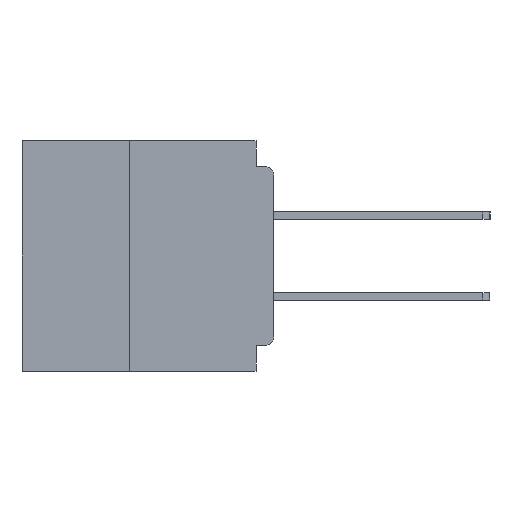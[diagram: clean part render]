
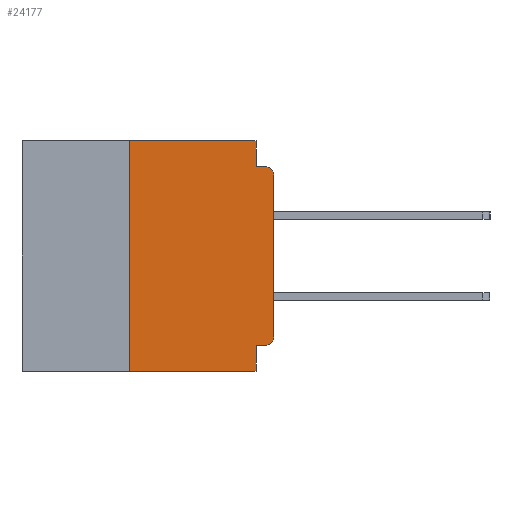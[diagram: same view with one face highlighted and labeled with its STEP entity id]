
A CAD part, left-side view. The second image highlights one B-rep face of the part: STEP entity #24177.
In plain terms, the highlighted planar face has unit normal (-1, 0, 0).
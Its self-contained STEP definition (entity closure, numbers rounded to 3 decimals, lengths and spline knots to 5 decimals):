
#228 = EDGE_CURVE ( 'NONE', #13836, #60963, #45011, .T. ) ;
#1067 = CARTESIAN_POINT ( 'NONE',  ( 0., 0.015, -0.34 ) ) ;
#1160 = ORIENTED_EDGE ( 'NONE', *, *, #29349, .F. ) ;
#1319 = CARTESIAN_POINT ( 'NONE',  ( 0., 0.25, -0.4 ) ) ;
#1442 = VERTEX_POINT ( 'NONE', #9127 ) ;
#1668 = LINE ( 'NONE', #40879, #40214 ) ;
#2097 = ORIENTED_EDGE ( 'NONE', *, *, #30204, .T. ) ;
#3158 = CARTESIAN_POINT ( 'NONE',  ( 0., 0., -0.355 ) ) ;
#3303 = ORIENTED_EDGE ( 'NONE', *, *, #56615, .F. ) ;
#4319 = CARTESIAN_POINT ( 'NONE',  ( 0., 0.031, 0. ) ) ;
#4534 = CIRCLE ( 'NONE', #47933, 0.015 ) ;
#5000 = VECTOR ( 'NONE', #17848, 39.37008 ) ;
#5638 = VERTEX_POINT ( 'NONE', #10580 ) ;
#6175 = DIRECTION ( 'NONE',  ( 0., 0., -1. ) ) ;
#6735 = CARTESIAN_POINT ( 'NONE',  ( 0., 0.437, -0.4 ) ) ;
#7118 = ORIENTED_EDGE ( 'NONE', *, *, #20436, .F. ) ;
#7853 = DIRECTION ( 'NONE',  ( 1., 0., 0. ) ) ;
#7890 = CARTESIAN_POINT ( 'NONE',  ( 0., 0., -0.045 ) ) ;
#8258 = CARTESIAN_POINT ( 'NONE',  ( 0., 0.031, 0. ) ) ;
#8943 = VECTOR ( 'NONE', #39429, 39.37008 ) ;
#9127 = CARTESIAN_POINT ( 'NONE',  ( 0., 0.031, -0.355 ) ) ;
#9786 = EDGE_CURVE ( 'NONE', #34087, #61449, #45298, .T. ) ;
#10580 = CARTESIAN_POINT ( 'NONE',  ( 0., 0., -0.34 ) ) ;
#10843 = DIRECTION ( 'NONE',  ( 0., 0., -1. ) ) ;
#11444 = DIRECTION ( 'NONE',  ( -1., 0., 0. ) ) ;
#13172 = EDGE_CURVE ( 'NONE', #60963, #28834, #20707, .T. ) ;
#13836 = VERTEX_POINT ( 'NONE', #59345 ) ;
#14243 = CARTESIAN_POINT ( 'NONE',  ( 0., 0.015, -0.045 ) ) ;
#17001 = VECTOR ( 'NONE', #42982, 39.37008 ) ;
#17848 = DIRECTION ( 'NONE',  ( 0., -1., 0. ) ) ;
#17987 = CARTESIAN_POINT ( 'NONE',  ( 0., 0.437, 0. ) ) ;
#19892 = CIRCLE ( 'NONE', #29870, 0.015 ) ;
#20436 = EDGE_CURVE ( 'NONE', #28834, #55717, #28709, .T. ) ;
#20707 = LINE ( 'NONE', #4319, #8943 ) ;
#21623 = CARTESIAN_POINT ( 'NONE',  ( 0., 0., 0. ) ) ;
#21842 = LINE ( 'NONE', #21623, #60128 ) ;
#22198 = EDGE_CURVE ( 'NONE', #32363, #55717, #19892, .T. ) ;
#23073 = CARTESIAN_POINT ( 'NONE',  ( 0., 0., -0.06 ) ) ;
#24177 = ADVANCED_FACE ( 'NONE', ( #63379 ), #38147, .F. ) ;
#26897 = DIRECTION ( 'NONE',  ( 0., -1., 0. ) ) ;
#28709 = LINE ( 'NONE', #7890, #17001 ) ;
#28834 = VERTEX_POINT ( 'NONE', #63838 ) ;
#29349 = EDGE_CURVE ( 'NONE', #38961, #1442, #44383, .T. ) ;
#29870 = AXIS2_PLACEMENT_3D ( 'NONE', #41478, #11444, #46488 ) ;
#30204 = EDGE_CURVE ( 'NONE', #38961, #5638, #4534, .T. ) ;
#31016 = VECTOR ( 'NONE', #38297, 39.37008 ) ;
#31783 = EDGE_LOOP ( 'NONE', ( #56810, #55645, #7118, #62825, #58824, #3303, #45698, #42251, #1160, #2097 ) ) ;
#31991 = VECTOR ( 'NONE', #26897, 39.37008 ) ;
#32114 = CARTESIAN_POINT ( 'NONE',  ( 0., 0.031, -0.4 ) ) ;
#32363 = VERTEX_POINT ( 'NONE', #23073 ) ;
#32985 = VECTOR ( 'NONE', #61302, 39.37008 ) ;
#33083 = CARTESIAN_POINT ( 'NONE',  ( 0., 0.437, 0. ) ) ;
#34087 = VERTEX_POINT ( 'NONE', #45841 ) ;
#36245 = DIRECTION ( 'NONE',  ( -1., 0., 0. ) ) ;
#37965 = AXIS2_PLACEMENT_3D ( 'NONE', #33083, #7853, #43161 ) ;
#38147 = PLANE ( 'NONE',  #37965 ) ;
#38297 = DIRECTION ( 'NONE',  ( 0., 1., 0. ) ) ;
#38961 = VERTEX_POINT ( 'NONE', #43491 ) ;
#39429 = DIRECTION ( 'NONE',  ( 0., 0., -1. ) ) ;
#40214 = VECTOR ( 'NONE', #10843, 39.37008 ) ;
#40879 = CARTESIAN_POINT ( 'NONE',  ( 0., 0.031, -0.4 ) ) ;
#41478 = CARTESIAN_POINT ( 'NONE',  ( 0., 0.015, -0.06 ) ) ;
#42251 = ORIENTED_EDGE ( 'NONE', *, *, #43575, .F. ) ;
#42982 = DIRECTION ( 'NONE',  ( 0., -1., 0. ) ) ;
#43161 = DIRECTION ( 'NONE',  ( 0., 0., -1. ) ) ;
#43491 = CARTESIAN_POINT ( 'NONE',  ( 0., 0.015, -0.355 ) ) ;
#43575 = EDGE_CURVE ( 'NONE', #1442, #61449, #1668, .T. ) ;
#44383 = LINE ( 'NONE', #3158, #31016 ) ;
#45011 = LINE ( 'NONE', #17987, #5000 ) ;
#45298 = LINE ( 'NONE', #6735, #31991 ) ;
#45698 = ORIENTED_EDGE ( 'NONE', *, *, #9786, .T. ) ;
#45841 = CARTESIAN_POINT ( 'NONE',  ( 0., 0.25, -0.4 ) ) ;
#46488 = DIRECTION ( 'NONE',  ( 0., 0., -1. ) ) ;
#47933 = AXIS2_PLACEMENT_3D ( 'NONE', #1067, #36245, #6175 ) ;
#49438 = LINE ( 'NONE', #1319, #32985 ) ;
#54316 = EDGE_CURVE ( 'NONE', #5638, #32363, #21842, .T. ) ;
#55645 = ORIENTED_EDGE ( 'NONE', *, *, #22198, .T. ) ;
#55717 = VERTEX_POINT ( 'NONE', #14243 ) ;
#56579 = DIRECTION ( 'NONE',  ( 0., 0., 1. ) ) ;
#56615 = EDGE_CURVE ( 'NONE', #34087, #13836, #49438, .T. ) ;
#56810 = ORIENTED_EDGE ( 'NONE', *, *, #54316, .T. ) ;
#58824 = ORIENTED_EDGE ( 'NONE', *, *, #228, .F. ) ;
#59345 = CARTESIAN_POINT ( 'NONE',  ( 0., 0.25, 0. ) ) ;
#60128 = VECTOR ( 'NONE', #56579, 39.37008 ) ;
#60963 = VERTEX_POINT ( 'NONE', #8258 ) ;
#61302 = DIRECTION ( 'NONE',  ( 0., 0., 1. ) ) ;
#61449 = VERTEX_POINT ( 'NONE', #32114 ) ;
#62825 = ORIENTED_EDGE ( 'NONE', *, *, #13172, .F. ) ;
#63379 = FACE_OUTER_BOUND ( 'NONE', #31783, .T. ) ;
#63838 = CARTESIAN_POINT ( 'NONE',  ( 0., 0.031, -0.045 ) ) ;
